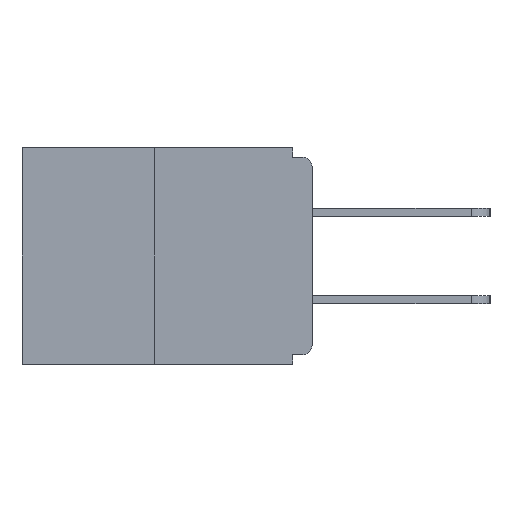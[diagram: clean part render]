
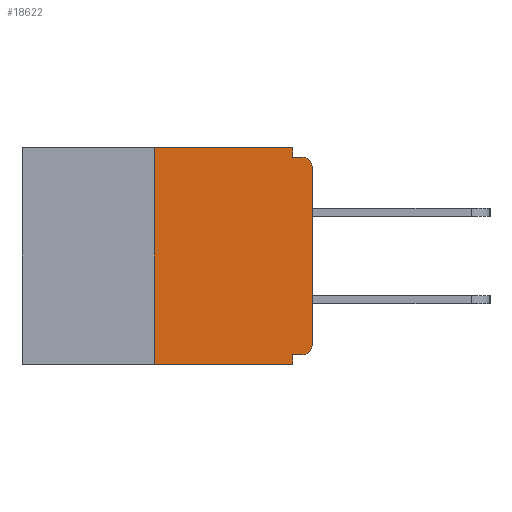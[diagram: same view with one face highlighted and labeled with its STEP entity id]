
A CAD part, left-side view. The second image highlights one B-rep face of the part: STEP entity #18622.
In plain terms, the highlighted planar face has unit normal (-1, 0, 0).
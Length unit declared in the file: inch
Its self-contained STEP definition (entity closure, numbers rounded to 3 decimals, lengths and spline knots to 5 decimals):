
#56 = CARTESIAN_POINT ( 'NONE',  ( 0., 0.031, -0.343 ) ) ;
#387 = VERTEX_POINT ( 'NONE', #22071 ) ;
#415 = CARTESIAN_POINT ( 'NONE',  ( 0., 0.015, -0.03 ) ) ;
#928 = DIRECTION ( 'NONE',  ( 1., 0., 0. ) ) ;
#992 = VECTOR ( 'NONE', #2796, 39.37008 ) ;
#1144 = ORIENTED_EDGE ( 'NONE', *, *, #16864, .T. ) ;
#1980 = DIRECTION ( 'NONE',  ( 0., -1., 0. ) ) ;
#2087 = CARTESIAN_POINT ( 'NONE',  ( 0., 0.031, -0.343 ) ) ;
#2381 = CARTESIAN_POINT ( 'NONE',  ( 0., 0.031, 0. ) ) ;
#2582 = VECTOR ( 'NONE', #5379, 39.37008 ) ;
#2796 = DIRECTION ( 'NONE',  ( 0., 0., 1. ) ) ;
#2993 = DIRECTION ( 'NONE',  ( 0., -1., 0. ) ) ;
#3019 = CARTESIAN_POINT ( 'NONE',  ( 0., 0.25, -0.343 ) ) ;
#3075 = VERTEX_POINT ( 'NONE', #2087 ) ;
#3814 = VECTOR ( 'NONE', #9194, 39.37008 ) ;
#4708 = DIRECTION ( 'NONE',  ( -1., 0., 0. ) ) ;
#4812 = CARTESIAN_POINT ( 'NONE',  ( 0., 0.46, 0. ) ) ;
#4823 = CARTESIAN_POINT ( 'NONE',  ( 0., 0.015, -0.015 ) ) ;
#5379 = DIRECTION ( 'NONE',  ( 0., 0., -1. ) ) ;
#5878 = CARTESIAN_POINT ( 'NONE',  ( 0., 0.031, -0.328 ) ) ;
#6302 = DIRECTION ( 'NONE',  ( 0., 0., -1. ) ) ;
#6601 = EDGE_CURVE ( 'NONE', #9216, #7485, #20611, .T. ) ;
#6787 = VERTEX_POINT ( 'NONE', #15771 ) ;
#6885 = VECTOR ( 'NONE', #22068, 39.37008 ) ;
#7197 = CARTESIAN_POINT ( 'NONE',  ( 0., 0.25, 0. ) ) ;
#7485 = VERTEX_POINT ( 'NONE', #2381 ) ;
#7674 = EDGE_CURVE ( 'NONE', #387, #6787, #13004, .T. ) ;
#8585 = EDGE_CURVE ( 'NONE', #23175, #3075, #9066, .T. ) ;
#9066 = LINE ( 'NONE', #56, #19307 ) ;
#9105 = EDGE_CURVE ( 'NONE', #18471, #9216, #9988, .T. ) ;
#9194 = DIRECTION ( 'NONE',  ( 0., 0., 1. ) ) ;
#9216 = VERTEX_POINT ( 'NONE', #15875 ) ;
#9534 = VECTOR ( 'NONE', #23556, 39.37008 ) ;
#9672 = ORIENTED_EDGE ( 'NONE', *, *, #22250, .F. ) ;
#9988 = LINE ( 'NONE', #7197, #3814 ) ;
#10256 = ORIENTED_EDGE ( 'NONE', *, *, #9105, .F. ) ;
#10656 = CARTESIAN_POINT ( 'NONE',  ( 0., 0.031, -0.015 ) ) ;
#10687 = LINE ( 'NONE', #11823, #12524 ) ;
#10726 = LINE ( 'NONE', #11760, #9534 ) ;
#11425 = ORIENTED_EDGE ( 'NONE', *, *, #12375, .T. ) ;
#11760 = CARTESIAN_POINT ( 'NONE',  ( 0., 0.46, -0.343 ) ) ;
#11823 = CARTESIAN_POINT ( 'NONE',  ( 0., 0., -0.015 ) ) ;
#11902 = ORIENTED_EDGE ( 'NONE', *, *, #8585, .F. ) ;
#12375 = EDGE_CURVE ( 'NONE', #6787, #14031, #15377, .T. ) ;
#12434 = ORIENTED_EDGE ( 'NONE', *, *, #7674, .T. ) ;
#12524 = VECTOR ( 'NONE', #1980, 39.37008 ) ;
#12608 = AXIS2_PLACEMENT_3D ( 'NONE', #4812, #928, #12735 ) ;
#12735 = DIRECTION ( 'NONE',  ( 0., 0., -1. ) ) ;
#12861 = EDGE_CURVE ( 'NONE', #24004, #14031, #10687, .T. ) ;
#13004 = LINE ( 'NONE', #20516, #992 ) ;
#13138 = ORIENTED_EDGE ( 'NONE', *, *, #6601, .F. ) ;
#13614 = EDGE_LOOP ( 'NONE', ( #13138, #10256, #20680, #11902, #17448, #1144, #12434, #11425, #13789, #9672 ) ) ;
#13758 = CARTESIAN_POINT ( 'NONE',  ( 0., 0., -0.328 ) ) ;
#13789 = ORIENTED_EDGE ( 'NONE', *, *, #12861, .F. ) ;
#14031 = VERTEX_POINT ( 'NONE', #4823 ) ;
#14250 = PLANE ( 'NONE',  #12608 ) ;
#14757 = AXIS2_PLACEMENT_3D ( 'NONE', #16845, #4708, #22687 ) ;
#15017 = EDGE_CURVE ( 'NONE', #18134, #23175, #23997, .T. ) ;
#15377 = CIRCLE ( 'NONE', #16211, 0.015 ) ;
#15627 = VECTOR ( 'NONE', #2993, 39.37008 ) ;
#15771 = CARTESIAN_POINT ( 'NONE',  ( 0., 0., -0.03 ) ) ;
#15875 = CARTESIAN_POINT ( 'NONE',  ( 0., 0.25, 0. ) ) ;
#16211 = AXIS2_PLACEMENT_3D ( 'NONE', #415, #22207, #6302 ) ;
#16588 = CARTESIAN_POINT ( 'NONE',  ( 0., 0.031, 0. ) ) ;
#16845 = CARTESIAN_POINT ( 'NONE',  ( 0., 0.015, -0.313 ) ) ;
#16864 = EDGE_CURVE ( 'NONE', #18134, #387, #17707, .T. ) ;
#17448 = ORIENTED_EDGE ( 'NONE', *, *, #15017, .F. ) ;
#17573 = DIRECTION ( 'NONE',  ( 0., 0., -1. ) ) ;
#17707 = CIRCLE ( 'NONE', #14757, 0.015 ) ;
#18134 = VERTEX_POINT ( 'NONE', #22518 ) ;
#18331 = EDGE_CURVE ( 'NONE', #18471, #3075, #10726, .T. ) ;
#18471 = VERTEX_POINT ( 'NONE', #3019 ) ;
#18622 = ADVANCED_FACE ( 'NONE', ( #24749 ), #14250, .F. ) ;
#19307 = VECTOR ( 'NONE', #17573, 39.37008 ) ;
#20516 = CARTESIAN_POINT ( 'NONE',  ( 0., 0., 0. ) ) ;
#20611 = LINE ( 'NONE', #20967, #15627 ) ;
#20680 = ORIENTED_EDGE ( 'NONE', *, *, #18331, .T. ) ;
#20967 = CARTESIAN_POINT ( 'NONE',  ( 0., 0.46, 0. ) ) ;
#22068 = DIRECTION ( 'NONE',  ( 0., 1., 0. ) ) ;
#22071 = CARTESIAN_POINT ( 'NONE',  ( 0., 0., -0.313 ) ) ;
#22207 = DIRECTION ( 'NONE',  ( -1., 0., 0. ) ) ;
#22250 = EDGE_CURVE ( 'NONE', #7485, #24004, #24048, .T. ) ;
#22518 = CARTESIAN_POINT ( 'NONE',  ( 0., 0.015, -0.328 ) ) ;
#22687 = DIRECTION ( 'NONE',  ( 0., 0., -1. ) ) ;
#23175 = VERTEX_POINT ( 'NONE', #5878 ) ;
#23556 = DIRECTION ( 'NONE',  ( 0., -1., 0. ) ) ;
#23997 = LINE ( 'NONE', #13758, #6885 ) ;
#24004 = VERTEX_POINT ( 'NONE', #10656 ) ;
#24048 = LINE ( 'NONE', #16588, #2582 ) ;
#24749 = FACE_OUTER_BOUND ( 'NONE', #13614, .T. ) ;
